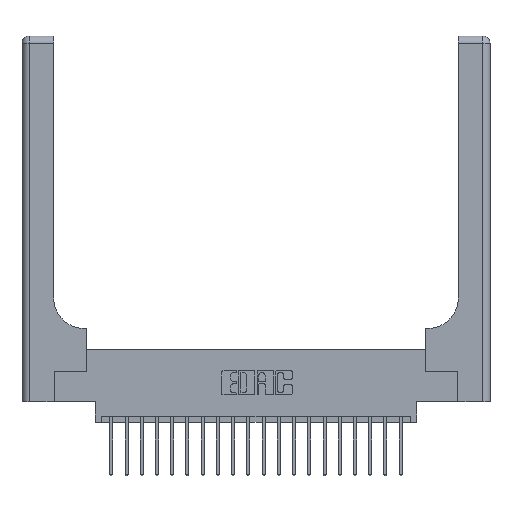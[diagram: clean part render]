
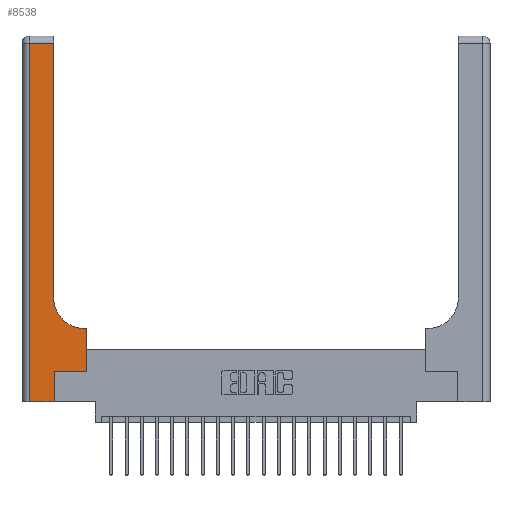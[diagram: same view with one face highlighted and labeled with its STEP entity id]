
A CAD part, top view. The second image highlights one B-rep face of the part: STEP entity #8538.
In plain terms, the highlighted planar face has unit normal (0, 0, 1).
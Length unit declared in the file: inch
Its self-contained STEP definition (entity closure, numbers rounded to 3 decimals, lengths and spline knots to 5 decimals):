
#364 = VECTOR ( 'NONE', #16207, 39.37008 ) ;
#414 = EDGE_CURVE ( 'NONE', #6909, #5621, #20013, .T. ) ;
#558 = EDGE_CURVE ( 'NONE', #17261, #10908, #9118, .T. ) ;
#723 = ORIENTED_EDGE ( 'NONE', *, *, #16016, .T. ) ;
#955 = CARTESIAN_POINT ( 'NONE',  ( 0.528, 0.25, 0.37 ) ) ;
#1117 = ORIENTED_EDGE ( 'NONE', *, *, #558, .T. ) ;
#2236 = CIRCLE ( 'NONE', #15424, 0.25 ) ;
#2590 = DIRECTION ( 'NONE',  ( 0., 1., 0. ) ) ;
#2607 = ORIENTED_EDGE ( 'NONE', *, *, #8193, .T. ) ;
#2994 = CARTESIAN_POINT ( 'NONE',  ( 0.26, 3., 0.37 ) ) ;
#3087 = VERTEX_POINT ( 'NONE', #17134 ) ;
#3304 = ORIENTED_EDGE ( 'NONE', *, *, #18266, .T. ) ;
#5576 = DIRECTION ( 'NONE',  ( 1., 0., 0. ) ) ;
#5621 = VERTEX_POINT ( 'NONE', #18445 ) ;
#6290 = DIRECTION ( 'NONE',  ( -1., 0., 0. ) ) ;
#6909 = VERTEX_POINT ( 'NONE', #7428 ) ;
#7133 = FACE_OUTER_BOUND ( 'NONE', #15735, .T. ) ;
#7428 = CARTESIAN_POINT ( 'NONE',  ( 0.06, 2.94, 0.37 ) ) ;
#7440 = LINE ( 'NONE', #17073, #11226 ) ;
#7809 = VECTOR ( 'NONE', #6290, 39.37008 ) ;
#7852 = VERTEX_POINT ( 'NONE', #16013 ) ;
#7916 = DIRECTION ( 'NONE',  ( 0., 0., -1. ) ) ;
#8193 = EDGE_CURVE ( 'NONE', #10908, #3087, #13808, .T. ) ;
#8322 = CARTESIAN_POINT ( 'NONE',  ( 0.265, 0., 0.37 ) ) ;
#8374 = ORIENTED_EDGE ( 'NONE', *, *, #15543, .T. ) ;
#8538 = ADVANCED_FACE ( 'NONE', ( #7133 ), #16282, .F. ) ;
#8604 = LINE ( 'NONE', #2994, #12410 ) ;
#9118 = LINE ( 'NONE', #8322, #17930 ) ;
#9721 = CARTESIAN_POINT ( 'NONE',  ( 0., 3., 0.37 ) ) ;
#9738 = CARTESIAN_POINT ( 'NONE',  ( 0.26, 0.85, 0.37 ) ) ;
#9836 = ORIENTED_EDGE ( 'NONE', *, *, #414, .T. ) ;
#10418 = CARTESIAN_POINT ( 'NONE',  ( 0.51, 0.6, 0.37 ) ) ;
#10695 = EDGE_CURVE ( 'NONE', #12786, #15454, #8604, .T. ) ;
#10908 = VERTEX_POINT ( 'NONE', #14998 ) ;
#11226 = VECTOR ( 'NONE', #5576, 39.37008 ) ;
#11346 = DIRECTION ( 'NONE',  ( -1., 0., 0. ) ) ;
#11900 = ORIENTED_EDGE ( 'NONE', *, *, #10695, .T. ) ;
#12103 = LINE ( 'NONE', #12773, #7809 ) ;
#12410 = VECTOR ( 'NONE', #14509, 39.37008 ) ;
#12773 = CARTESIAN_POINT ( 'NONE',  ( 0., 2.94, 0.37 ) ) ;
#12786 = VERTEX_POINT ( 'NONE', #9738 ) ;
#13415 = DIRECTION ( 'NONE',  ( 1., 0., 0. ) ) ;
#13522 = VECTOR ( 'NONE', #2590, 39.37008 ) ;
#13808 = LINE ( 'NONE', #20114, #17730 ) ;
#14039 = LINE ( 'NONE', #955, #13522 ) ;
#14509 = DIRECTION ( 'NONE',  ( 0., 1., 0. ) ) ;
#14998 = CARTESIAN_POINT ( 'NONE',  ( 0.265, 0.25, 0.37 ) ) ;
#15424 = AXIS2_PLACEMENT_3D ( 'NONE', #17798, #7916, #19487 ) ;
#15454 = VERTEX_POINT ( 'NONE', #18473 ) ;
#15543 = EDGE_CURVE ( 'NONE', #5621, #17261, #7440, .T. ) ;
#15735 = EDGE_LOOP ( 'NONE', ( #11900, #21195, #9836, #8374, #1117, #2607, #723, #3304, #20129 ) ) ;
#15833 = EDGE_CURVE ( 'NONE', #21216, #12786, #2236, .T. ) ;
#15993 = DIRECTION ( 'NONE',  ( 0., -1., 0. ) ) ;
#16013 = CARTESIAN_POINT ( 'NONE',  ( 0.528, 0.6, 0.37 ) ) ;
#16016 = EDGE_CURVE ( 'NONE', #3087, #7852, #14039, .T. ) ;
#16070 = VECTOR ( 'NONE', #15993, 39.37008 ) ;
#16207 = DIRECTION ( 'NONE',  ( -1., 0., 0. ) ) ;
#16282 = PLANE ( 'NONE',  #21137 ) ;
#16520 = DIRECTION ( 'NONE',  ( 0., 1., 0. ) ) ;
#17073 = CARTESIAN_POINT ( 'NONE',  ( 0., 0., 0.37 ) ) ;
#17134 = CARTESIAN_POINT ( 'NONE',  ( 0.528, 0.25, 0.37 ) ) ;
#17261 = VERTEX_POINT ( 'NONE', #18387 ) ;
#17712 = CARTESIAN_POINT ( 'NONE',  ( 0.06, 3., 0.37 ) ) ;
#17730 = VECTOR ( 'NONE', #13415, 39.37008 ) ;
#17798 = CARTESIAN_POINT ( 'NONE',  ( 0.51, 0.85, 0.37 ) ) ;
#17910 = LINE ( 'NONE', #19523, #364 ) ;
#17930 = VECTOR ( 'NONE', #16520, 39.37008 ) ;
#18266 = EDGE_CURVE ( 'NONE', #7852, #21216, #17910, .T. ) ;
#18387 = CARTESIAN_POINT ( 'NONE',  ( 0.265, 0., 0.37 ) ) ;
#18445 = CARTESIAN_POINT ( 'NONE',  ( 0.06, 0., 0.37 ) ) ;
#18473 = CARTESIAN_POINT ( 'NONE',  ( 0.26, 2.94, 0.37 ) ) ;
#19487 = DIRECTION ( 'NONE',  ( 1., 0., 0. ) ) ;
#19523 = CARTESIAN_POINT ( 'NONE',  ( 0.26, 0.6, 0.37 ) ) ;
#19634 = EDGE_CURVE ( 'NONE', #15454, #6909, #12103, .T. ) ;
#20013 = LINE ( 'NONE', #17712, #16070 ) ;
#20114 = CARTESIAN_POINT ( 'NONE',  ( 0.265, 0.25, 0.37 ) ) ;
#20129 = ORIENTED_EDGE ( 'NONE', *, *, #15833, .T. ) ;
#21137 = AXIS2_PLACEMENT_3D ( 'NONE', #9721, #21324, #11346 ) ;
#21195 = ORIENTED_EDGE ( 'NONE', *, *, #19634, .T. ) ;
#21216 = VERTEX_POINT ( 'NONE', #10418 ) ;
#21324 = DIRECTION ( 'NONE',  ( 0., 0., -1. ) ) ;
